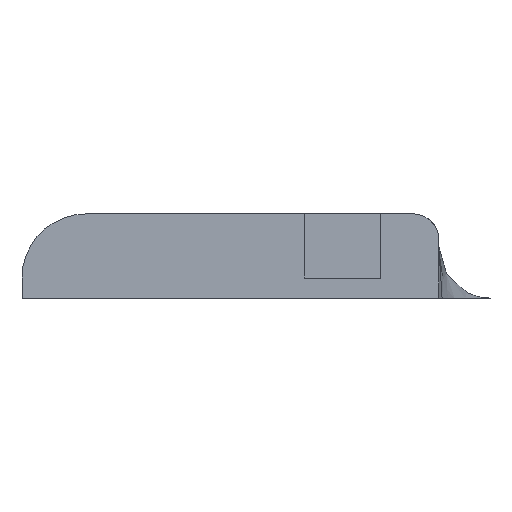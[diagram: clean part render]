
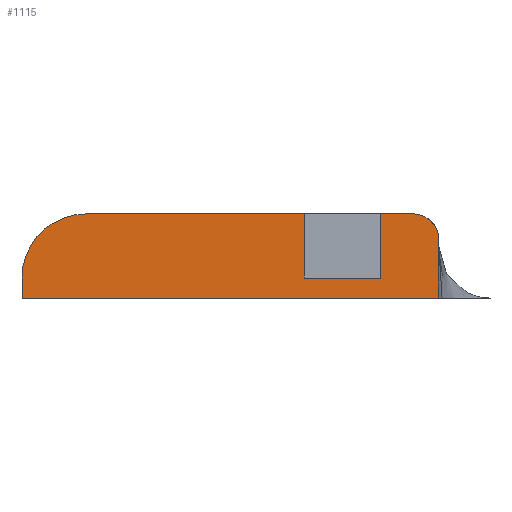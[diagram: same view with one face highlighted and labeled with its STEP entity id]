
A CAD part, left-side view. The second image highlights one B-rep face of the part: STEP entity #1115.
In plain terms, the highlighted planar face has unit normal (-1, 0, 0).
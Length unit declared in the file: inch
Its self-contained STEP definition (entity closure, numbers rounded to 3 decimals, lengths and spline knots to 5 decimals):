
#2 = DIRECTION ( 'NONE',  ( 0., -1., 0. ) ) ;
#7 = AXIS2_PLACEMENT_3D ( 'NONE', #1166, #951, #786 ) ;
#20 = CARTESIAN_POINT ( 'NONE',  ( 3.70038, -1.71568, 0.65223 ) ) ;
#24 = VECTOR ( 'NONE', #643, 39.37008 ) ;
#46 = CARTESIAN_POINT ( 'NONE',  ( 3.70038, -1.38086, 0.53412 ) ) ;
#67 = LINE ( 'NONE', #245, #24 ) ;
#90 = ORIENTED_EDGE ( 'NONE', *, *, #629, .T. ) ;
#91 = VERTEX_POINT ( 'NONE', #241 ) ;
#95 = VECTOR ( 'NONE', #948, 39.37008 ) ;
#113 = CARTESIAN_POINT ( 'NONE',  ( 3.70038, -0.71157, 0.53412 ) ) ;
#115 = VERTEX_POINT ( 'NONE', #1037 ) ;
#122 = LINE ( 'NONE', #844, #95 ) ;
#123 = DIRECTION ( 'NONE',  ( 0., 1., 0. ) ) ;
#144 = DIRECTION ( 'NONE',  ( 0., 0., 1. ) ) ;
#154 = CARTESIAN_POINT ( 'NONE',  ( 3.70038, -1.61708, 0.53412 ) ) ;
#160 = ORIENTED_EDGE ( 'NONE', *, *, #612, .T. ) ;
#185 = VERTEX_POINT ( 'NONE', #949 ) ;
#190 = CARTESIAN_POINT ( 'NONE',  ( 3.70038, -1.61708, 0.73097 ) ) ;
#216 = EDGE_LOOP ( 'NONE', ( #647, #609, #816, #90, #1128, #470, #1082, #1064, #1177, #160, #326 ) ) ;
#217 = DIRECTION ( 'NONE',  ( 0., 1., 0. ) ) ;
#241 = CARTESIAN_POINT ( 'NONE',  ( 3.70038, -1.79442, 0.65223 ) ) ;
#245 = CARTESIAN_POINT ( 'NONE',  ( 3.70038, -1.38086, 0.73097 ) ) ;
#276 = FACE_OUTER_BOUND ( 'NONE', #216, .T. ) ;
#294 = AXIS2_PLACEMENT_3D ( 'NONE', #20, #714, #123 ) ;
#301 = AXIS2_PLACEMENT_3D ( 'NONE', #113, #810, #217 ) ;
#317 = LINE ( 'NONE', #343, #1088 ) ;
#326 = ORIENTED_EDGE ( 'NONE', *, *, #725, .F. ) ;
#338 = DIRECTION ( 'NONE',  ( 0., 0., 1. ) ) ;
#343 = CARTESIAN_POINT ( 'NONE',  ( 3.70038, -1.61708, 0. ) ) ;
#349 = VERTEX_POINT ( 'NONE', #963 ) ;
#358 = VECTOR ( 'NONE', #338, 39.37008 ) ;
#392 = VECTOR ( 'NONE', #937, 39.37008 ) ;
#409 = VERTEX_POINT ( 'NONE', #548 ) ;
#432 = CARTESIAN_POINT ( 'NONE',  ( 3.70038, -0.51472, -0.70907 ) ) ;
#437 = VERTEX_POINT ( 'NONE', #154 ) ;
#440 = DIRECTION ( 'NONE',  ( 0., 0., -1. ) ) ;
#470 = ORIENTED_EDGE ( 'NONE', *, *, #748, .T. ) ;
#484 = LINE ( 'NONE', #924, #712 ) ;
#486 = CARTESIAN_POINT ( 'NONE',  ( 3.70038, -1.38086, 0.53412 ) ) ;
#548 = CARTESIAN_POINT ( 'NONE',  ( 3.70038, -1.38086, 0.73097 ) ) ;
#550 = VERTEX_POINT ( 'NONE', #983 ) ;
#559 = VECTOR ( 'NONE', #1126, 39.37008 ) ;
#582 = VECTOR ( 'NONE', #2, 39.37008 ) ;
#585 = EDGE_CURVE ( 'NONE', #1234, #550, #1099, .T. ) ;
#595 = LINE ( 'NONE', #46, #559 ) ;
#599 = CARTESIAN_POINT ( 'NONE',  ( 3.70038, 1.32551, 0.47244 ) ) ;
#609 = ORIENTED_EDGE ( 'NONE', *, *, #733, .T. ) ;
#611 = VECTOR ( 'NONE', #144, 39.37008 ) ;
#612 = EDGE_CURVE ( 'NONE', #851, #349, #809, .T. ) ;
#623 = CARTESIAN_POINT ( 'NONE',  ( 3.70038, -0.71157, 0.73097 ) ) ;
#629 = EDGE_CURVE ( 'NONE', #91, #115, #783, .T. ) ;
#643 = DIRECTION ( 'NONE',  ( 0., 0., -1. ) ) ;
#647 = ORIENTED_EDGE ( 'NONE', *, *, #585, .T. ) ;
#654 = LINE ( 'NONE', #432, #358 ) ;
#683 = EDGE_CURVE ( 'NONE', #409, #851, #484, .T. ) ;
#685 = PLANE ( 'NONE',  #7 ) ;
#712 = VECTOR ( 'NONE', #724, 39.37008 ) ;
#714 = DIRECTION ( 'NONE',  ( -1., 0., 0. ) ) ;
#716 = EDGE_CURVE ( 'NONE', #115, #1165, #1187, .T. ) ;
#724 = DIRECTION ( 'NONE',  ( 0., 1., 0. ) ) ;
#725 = EDGE_CURVE ( 'NONE', #1234, #349, #654, .T. ) ;
#733 = EDGE_CURVE ( 'NONE', #550, #185, #861, .T. ) ;
#740 = CARTESIAN_POINT ( 'NONE',  ( 3.70038, -1.79442, -1.63124 ) ) ;
#745 = EDGE_CURVE ( 'NONE', #91, #185, #122, .T. ) ;
#748 = EDGE_CURVE ( 'NONE', #1165, #437, #317, .T. ) ;
#758 = EDGE_CURVE ( 'NONE', #1183, #437, #595, .T. ) ;
#765 = EDGE_CURVE ( 'NONE', #409, #1183, #67, .T. ) ;
#783 = CIRCLE ( 'NONE', #294, 0.07874 ) ;
#786 = DIRECTION ( 'NONE',  ( 0., 1., 0. ) ) ;
#809 = CIRCLE ( 'NONE', #301, 0.19685 ) ;
#810 = DIRECTION ( 'NONE',  ( -1., 0., 0. ) ) ;
#816 = ORIENTED_EDGE ( 'NONE', *, *, #745, .F. ) ;
#844 = CARTESIAN_POINT ( 'NONE',  ( 3.70038, -1.79442, -1.11943 ) ) ;
#851 = VERTEX_POINT ( 'NONE', #623 ) ;
#861 = LINE ( 'NONE', #740, #611 ) ;
#924 = CARTESIAN_POINT ( 'NONE',  ( 3.70038, -0.47716, 0.73097 ) ) ;
#937 = DIRECTION ( 'NONE',  ( 0., 1., 0. ) ) ;
#948 = DIRECTION ( 'NONE',  ( 0., 0., -1. ) ) ;
#949 = CARTESIAN_POINT ( 'NONE',  ( 3.70038, -1.79442, 0.62992 ) ) ;
#951 = DIRECTION ( 'NONE',  ( 1., 0., 0. ) ) ;
#963 = CARTESIAN_POINT ( 'NONE',  ( 3.70038, -0.51472, 0.53412 ) ) ;
#983 = CARTESIAN_POINT ( 'NONE',  ( 3.70038, -1.79442, 0.47244 ) ) ;
#1001 = CARTESIAN_POINT ( 'NONE',  ( 3.70038, -0.51472, 0.47244 ) ) ;
#1024 = CARTESIAN_POINT ( 'NONE',  ( 3.70038, -0.47716, 0.73097 ) ) ;
#1037 = CARTESIAN_POINT ( 'NONE',  ( 3.70038, -1.71568, 0.73097 ) ) ;
#1064 = ORIENTED_EDGE ( 'NONE', *, *, #765, .F. ) ;
#1082 = ORIENTED_EDGE ( 'NONE', *, *, #758, .F. ) ;
#1088 = VECTOR ( 'NONE', #440, 39.37008 ) ;
#1099 = LINE ( 'NONE', #599, #582 ) ;
#1115 = ADVANCED_FACE ( 'NONE', ( #276 ), #685, .F. ) ;
#1126 = DIRECTION ( 'NONE',  ( 0., -1., 0. ) ) ;
#1128 = ORIENTED_EDGE ( 'NONE', *, *, #716, .T. ) ;
#1165 = VERTEX_POINT ( 'NONE', #190 ) ;
#1166 = CARTESIAN_POINT ( 'NONE',  ( 3.70038, 1.01705, 0.74273 ) ) ;
#1177 = ORIENTED_EDGE ( 'NONE', *, *, #683, .T. ) ;
#1183 = VERTEX_POINT ( 'NONE', #486 ) ;
#1187 = LINE ( 'NONE', #1024, #392 ) ;
#1234 = VERTEX_POINT ( 'NONE', #1001 ) ;
